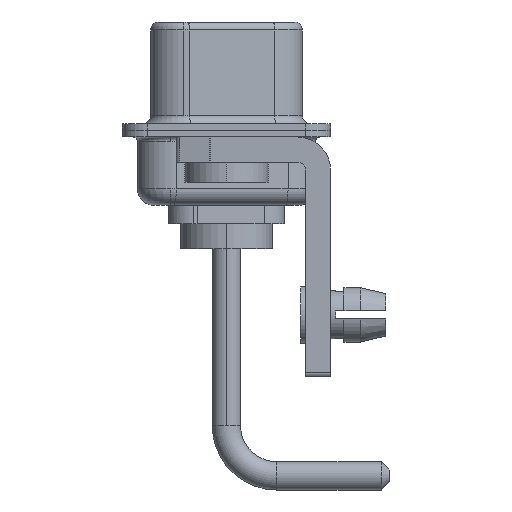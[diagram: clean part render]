
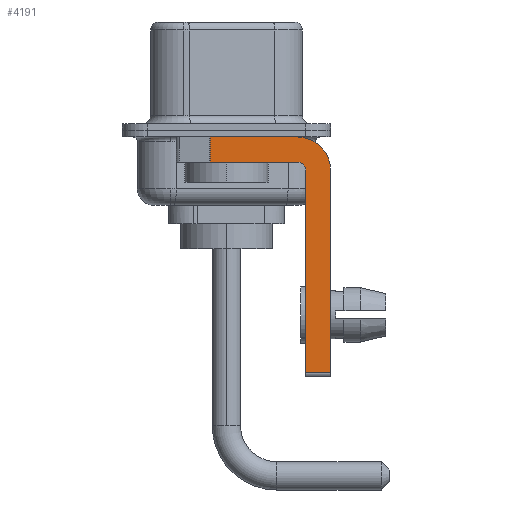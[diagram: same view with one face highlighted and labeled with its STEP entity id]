
A CAD part, left-side view. The second image highlights one B-rep face of the part: STEP entity #4191.
In plain terms, the highlighted planar face has unit normal (-1, 0, 0).
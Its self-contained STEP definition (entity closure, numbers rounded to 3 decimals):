
#172 = DIRECTION ( 'NONE',  ( 0., 1., 0. ) ) ;
#603 = LINE ( 'NONE', #13379, #7623 ) ;
#688 = CARTESIAN_POINT ( 'NONE',  ( -2.9, -4.25, -1.9 ) ) ;
#698 = EDGE_CURVE ( 'NONE', #17914, #14691, #16311, .T. ) ;
#705 = ORIENTED_EDGE ( 'NONE', *, *, #7997, .T. ) ;
#1648 = DIRECTION ( 'NONE',  ( 0., 0., 1. ) ) ;
#1666 = CARTESIAN_POINT ( 'NONE',  ( -2.9, 0.978, -0.4 ) ) ;
#2843 = CARTESIAN_POINT ( 'NONE',  ( -2.9, 0.978, -1.9 ) ) ;
#2994 = CARTESIAN_POINT ( 'NONE',  ( -2.9, -4.75, -14.8 ) ) ;
#3098 = DIRECTION ( 'NONE',  ( 0., -1., 0. ) ) ;
#3448 = VECTOR ( 'NONE', #8838, 1000. ) ;
#3821 = DIRECTION ( 'NONE',  ( 0., 0., -1. ) ) ;
#4026 = EDGE_CURVE ( 'NONE', #7166, #13809, #16019, .T. ) ;
#4125 = DIRECTION ( 'NONE',  ( 0., 0., -1. ) ) ;
#4191 = ADVANCED_FACE ( 'NONE', ( #17910 ), #7701, .F. ) ;
#4945 = DIRECTION ( 'NONE',  ( 1., 0., 0. ) ) ;
#4994 = EDGE_CURVE ( 'NONE', #13809, #11318, #12548, .T. ) ;
#5825 = EDGE_CURVE ( 'NONE', #14691, #12091, #18201, .T. ) ;
#6550 = CARTESIAN_POINT ( 'NONE',  ( -2.9, -4.25, -2.4 ) ) ;
#7057 = LINE ( 'NONE', #13030, #10037 ) ;
#7166 = VERTEX_POINT ( 'NONE', #16337 ) ;
#7312 = EDGE_LOOP ( 'NONE', ( #10121, #8237, #17799, #12346, #18123, #705, #18141, #18099 ) ) ;
#7353 = CARTESIAN_POINT ( 'NONE',  ( -2.9, -6.25, -2.4 ) ) ;
#7378 = CARTESIAN_POINT ( 'NONE',  ( -2.9, -4.25, -2.4 ) ) ;
#7623 = VECTOR ( 'NONE', #17791, 1000. ) ;
#7701 = PLANE ( 'NONE',  #8558 ) ;
#7911 = LINE ( 'NONE', #17441, #18367 ) ;
#7997 = EDGE_CURVE ( 'NONE', #7166, #12091, #603, .T. ) ;
#8157 = AXIS2_PLACEMENT_3D ( 'NONE', #11338, #11426, #4125 ) ;
#8237 = ORIENTED_EDGE ( 'NONE', *, *, #17745, .T. ) ;
#8558 = AXIS2_PLACEMENT_3D ( 'NONE', #6550, #4945, #13676 ) ;
#8574 = DIRECTION ( 'NONE',  ( 0., 0., -1. ) ) ;
#8838 = DIRECTION ( 'NONE',  ( 0., 0., 1. ) ) ;
#8883 = AXIS2_PLACEMENT_3D ( 'NONE', #7378, #17307, #1648 ) ;
#9290 = CARTESIAN_POINT ( 'NONE',  ( -2.9, -6.25, -14.55 ) ) ;
#10037 = VECTOR ( 'NONE', #3098, 1000. ) ;
#10084 = EDGE_CURVE ( 'NONE', #13366, #17914, #7057, .T. ) ;
#10121 = ORIENTED_EDGE ( 'NONE', *, *, #10084, .F. ) ;
#11318 = VERTEX_POINT ( 'NONE', #688 ) ;
#11338 = CARTESIAN_POINT ( 'NONE',  ( -2.9, -4.25, -2.4 ) ) ;
#11426 = DIRECTION ( 'NONE',  ( 1., 0., 0. ) ) ;
#11435 = LINE ( 'NONE', #2843, #13050 ) ;
#11822 = CARTESIAN_POINT ( 'NONE',  ( -2.9, -4.75, -2.4 ) ) ;
#11960 = VECTOR ( 'NONE', #3821, 1000. ) ;
#12091 = VERTEX_POINT ( 'NONE', #9290 ) ;
#12346 = ORIENTED_EDGE ( 'NONE', *, *, #4994, .F. ) ;
#12548 = CIRCLE ( 'NONE', #8883, 0.5 ) ;
#12921 = EDGE_CURVE ( 'NONE', #11318, #17785, #7911, .T. ) ;
#13030 = CARTESIAN_POINT ( 'NONE',  ( -2.9, 3., -0.4 ) ) ;
#13050 = VECTOR ( 'NONE', #8574, 1000. ) ;
#13241 = CARTESIAN_POINT ( 'NONE',  ( -2.9, 0.978, -1.9 ) ) ;
#13366 = VERTEX_POINT ( 'NONE', #1666 ) ;
#13379 = CARTESIAN_POINT ( 'NONE',  ( -2.9, -4.25, -14.55 ) ) ;
#13676 = DIRECTION ( 'NONE',  ( 0., 0., -1. ) ) ;
#13809 = VERTEX_POINT ( 'NONE', #11822 ) ;
#14691 = VERTEX_POINT ( 'NONE', #7353 ) ;
#15470 = CARTESIAN_POINT ( 'NONE',  ( -2.9, -4.25, -0.4 ) ) ;
#16019 = LINE ( 'NONE', #2994, #3448 ) ;
#16311 = CIRCLE ( 'NONE', #8157, 2. ) ;
#16337 = CARTESIAN_POINT ( 'NONE',  ( -2.9, -4.75, -14.55 ) ) ;
#16765 = CARTESIAN_POINT ( 'NONE',  ( -2.9, -6.25, -2.4 ) ) ;
#17307 = DIRECTION ( 'NONE',  ( -1., 0., 0. ) ) ;
#17441 = CARTESIAN_POINT ( 'NONE',  ( -2.9, -4.25, -1.9 ) ) ;
#17745 = EDGE_CURVE ( 'NONE', #13366, #17785, #11435, .T. ) ;
#17785 = VERTEX_POINT ( 'NONE', #13241 ) ;
#17791 = DIRECTION ( 'NONE',  ( 0., -1., 0. ) ) ;
#17799 = ORIENTED_EDGE ( 'NONE', *, *, #12921, .F. ) ;
#17910 = FACE_OUTER_BOUND ( 'NONE', #7312, .T. ) ;
#17914 = VERTEX_POINT ( 'NONE', #15470 ) ;
#18099 = ORIENTED_EDGE ( 'NONE', *, *, #698, .F. ) ;
#18123 = ORIENTED_EDGE ( 'NONE', *, *, #4026, .F. ) ;
#18141 = ORIENTED_EDGE ( 'NONE', *, *, #5825, .F. ) ;
#18201 = LINE ( 'NONE', #16765, #11960 ) ;
#18367 = VECTOR ( 'NONE', #172, 1000. ) ;
